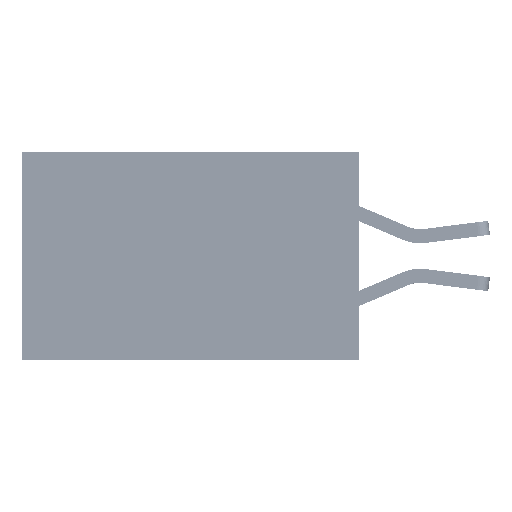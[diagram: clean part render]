
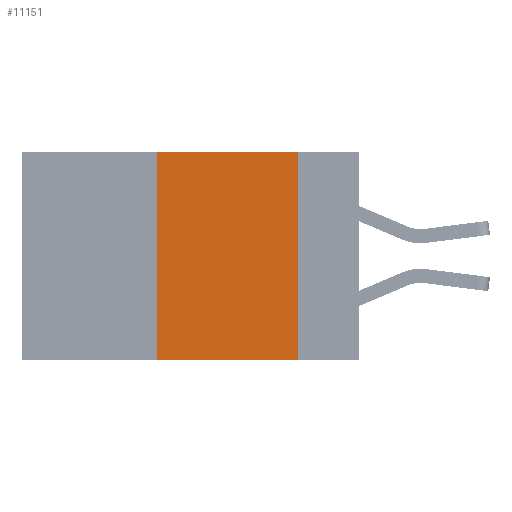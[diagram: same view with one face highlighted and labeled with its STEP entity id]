
A CAD part, left-side view. The second image highlights one B-rep face of the part: STEP entity #11151.
In plain terms, the highlighted planar face has unit normal (-1, 0, 0).
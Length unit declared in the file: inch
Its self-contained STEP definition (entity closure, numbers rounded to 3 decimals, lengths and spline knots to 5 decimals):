
#704 = LINE ( 'NONE', #34142, #33720 ) ;
#860 = AXIS2_PLACEMENT_3D ( 'NONE', #35558, #35192, #26925 ) ;
#1493 = ORIENTED_EDGE ( 'NONE', *, *, #35174, .T. ) ;
#1524 = VECTOR ( 'NONE', #17480, 39.37008 ) ;
#1636 = CARTESIAN_POINT ( 'NONE',  ( 0., 0.36, 0. ) ) ;
#1697 = EDGE_CURVE ( 'NONE', #17830, #14534, #704, .T. ) ;
#2631 = LINE ( 'NONE', #36820, #1524 ) ;
#4837 = ORIENTED_EDGE ( 'NONE', *, *, #1697, .F. ) ;
#4973 = ORIENTED_EDGE ( 'NONE', *, *, #28312, .F. ) ;
#7060 = VECTOR ( 'NONE', #30361, 39.37008 ) ;
#7144 = VECTOR ( 'NONE', #28018, 39.37008 ) ;
#10564 = LINE ( 'NONE', #33459, #7144 ) ;
#11151 = ADVANCED_FACE ( 'NONE', ( #29731 ), #23561, .F. ) ;
#12401 = CARTESIAN_POINT ( 'NONE',  ( 0., 0.36, 0. ) ) ;
#14534 = VERTEX_POINT ( 'NONE', #23145 ) ;
#15689 = EDGE_LOOP ( 'NONE', ( #4837, #4973, #28896, #1493 ) ) ;
#17480 = DIRECTION ( 'NONE',  ( 0., -1., 0. ) ) ;
#17830 = VERTEX_POINT ( 'NONE', #18036 ) ;
#17837 = VERTEX_POINT ( 'NONE', #12401 ) ;
#18036 = CARTESIAN_POINT ( 'NONE',  ( 0., 0.11, 0. ) ) ;
#18930 = LINE ( 'NONE', #1636, #7060 ) ;
#19890 = DIRECTION ( 'NONE',  ( 0., 0., -1. ) ) ;
#21412 = VERTEX_POINT ( 'NONE', #24091 ) ;
#23145 = CARTESIAN_POINT ( 'NONE',  ( 0., 0.11, -0.37 ) ) ;
#23561 = PLANE ( 'NONE',  #860 ) ;
#24091 = CARTESIAN_POINT ( 'NONE',  ( 0., 0.36, -0.37 ) ) ;
#26925 = DIRECTION ( 'NONE',  ( 0., 0., -1. ) ) ;
#28018 = DIRECTION ( 'NONE',  ( 0., -1., 0. ) ) ;
#28312 = EDGE_CURVE ( 'NONE', #17837, #17830, #2631, .T. ) ;
#28896 = ORIENTED_EDGE ( 'NONE', *, *, #33342, .F. ) ;
#29731 = FACE_OUTER_BOUND ( 'NONE', #15689, .T. ) ;
#30361 = DIRECTION ( 'NONE',  ( 0., 0., 1. ) ) ;
#33342 = EDGE_CURVE ( 'NONE', #21412, #17837, #18930, .T. ) ;
#33459 = CARTESIAN_POINT ( 'NONE',  ( 0., 0.6, -0.37 ) ) ;
#33720 = VECTOR ( 'NONE', #19890, 39.37008 ) ;
#34142 = CARTESIAN_POINT ( 'NONE',  ( 0., 0.11, 0. ) ) ;
#35174 = EDGE_CURVE ( 'NONE', #21412, #14534, #10564, .T. ) ;
#35192 = DIRECTION ( 'NONE',  ( 1., 0., 0. ) ) ;
#35558 = CARTESIAN_POINT ( 'NONE',  ( 0., 0.6, 0. ) ) ;
#36820 = CARTESIAN_POINT ( 'NONE',  ( 0., 0.6, 0. ) ) ;
